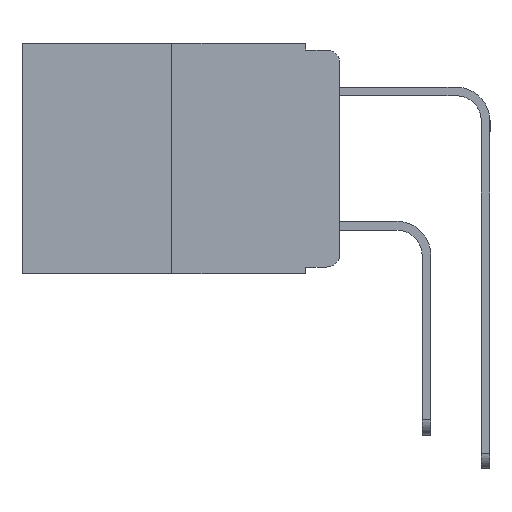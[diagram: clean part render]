
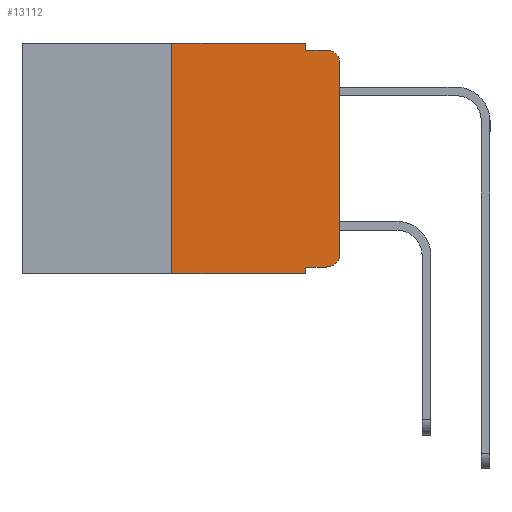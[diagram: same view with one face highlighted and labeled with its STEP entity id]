
A CAD part, left-side view. The second image highlights one B-rep face of the part: STEP entity #13112.
In plain terms, the highlighted planar face has unit normal (-1, 0, 0).
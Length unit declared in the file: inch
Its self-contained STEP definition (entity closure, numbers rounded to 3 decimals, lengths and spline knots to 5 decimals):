
#239 = VERTEX_POINT ( 'NONE', #8575 ) ;
#1704 = VERTEX_POINT ( 'NONE', #5237 ) ;
#1917 = VERTEX_POINT ( 'NONE', #10262 ) ;
#2383 = VECTOR ( 'NONE', #9094, 39.37008 ) ;
#2696 = ORIENTED_EDGE ( 'NONE', *, *, #4232, .T. ) ;
#3039 = LINE ( 'NONE', #15626, #9622 ) ;
#3083 = EDGE_CURVE ( 'NONE', #10547, #7417, #3039, .T. ) ;
#3260 = ORIENTED_EDGE ( 'NONE', *, *, #15916, .T. ) ;
#3425 = ORIENTED_EDGE ( 'NONE', *, *, #4683, .T. ) ;
#3644 = DIRECTION ( 'NONE',  ( 1., 0., 0. ) ) ;
#3712 = VERTEX_POINT ( 'NONE', #8653 ) ;
#3813 = EDGE_CURVE ( 'NONE', #7417, #6223, #8644, .T. ) ;
#3846 = CARTESIAN_POINT ( 'NONE',  ( 0., 0.473, -0.343 ) ) ;
#4232 = EDGE_CURVE ( 'NONE', #1704, #3712, #5195, .T. ) ;
#4366 = CIRCLE ( 'NONE', #16065, 0.02 ) ;
#4436 = CARTESIAN_POINT ( 'NONE',  ( 0., 0.051, 0. ) ) ;
#4580 = VECTOR ( 'NONE', #11531, 39.37008 ) ;
#4683 = EDGE_CURVE ( 'NONE', #10547, #239, #14860, .T. ) ;
#4753 = EDGE_CURVE ( 'NONE', #15833, #10341, #4366, .T. ) ;
#4819 = CIRCLE ( 'NONE', #9872, 0.02 ) ;
#5162 = CARTESIAN_POINT ( 'NONE',  ( 0., 0.02, -0.313 ) ) ;
#5195 = LINE ( 'NONE', #8244, #8019 ) ;
#5237 = CARTESIAN_POINT ( 'NONE',  ( 0., 0.051, -0.333 ) ) ;
#5358 = AXIS2_PLACEMENT_3D ( 'NONE', #11033, #3644, #12258 ) ;
#5512 = DIRECTION ( 'NONE',  ( 0., 0., -1. ) ) ;
#5885 = VECTOR ( 'NONE', #14178, 39.37008 ) ;
#5941 = EDGE_CURVE ( 'NONE', #1704, #239, #6253, .T. ) ;
#6223 = VERTEX_POINT ( 'NONE', #15981 ) ;
#6253 = LINE ( 'NONE', #4436, #5885 ) ;
#6355 = DIRECTION ( 'NONE',  ( 0., 0., -1. ) ) ;
#6383 = DIRECTION ( 'NONE',  ( -1., 0., 0. ) ) ;
#6387 = VECTOR ( 'NONE', #7710, 39.37008 ) ;
#6838 = CARTESIAN_POINT ( 'NONE',  ( 0., 0.02, -0.03 ) ) ;
#7074 = ORIENTED_EDGE ( 'NONE', *, *, #3813, .F. ) ;
#7205 = ORIENTED_EDGE ( 'NONE', *, *, #13690, .F. ) ;
#7300 = DIRECTION ( 'NONE',  ( 0., 0., 1. ) ) ;
#7417 = VERTEX_POINT ( 'NONE', #10091 ) ;
#7422 = EDGE_CURVE ( 'NONE', #1917, #10341, #16097, .T. ) ;
#7710 = DIRECTION ( 'NONE',  ( 0., -1., 0. ) ) ;
#8019 = VECTOR ( 'NONE', #10734, 39.37008 ) ;
#8244 = CARTESIAN_POINT ( 'NONE',  ( 0., 0.051, -0.333 ) ) ;
#8575 = CARTESIAN_POINT ( 'NONE',  ( 0., 0.051, -0.343 ) ) ;
#8619 = LINE ( 'NONE', #9923, #14722 ) ;
#8644 = LINE ( 'NONE', #14735, #2383 ) ;
#8653 = CARTESIAN_POINT ( 'NONE',  ( 0., 0.02, -0.333 ) ) ;
#8747 = DIRECTION ( 'NONE',  ( 0., 0., 1. ) ) ;
#9083 = CARTESIAN_POINT ( 'NONE',  ( 0., 0.051, 0. ) ) ;
#9094 = DIRECTION ( 'NONE',  ( 0., -1., 0. ) ) ;
#9380 = VERTEX_POINT ( 'NONE', #12667 ) ;
#9533 = VECTOR ( 'NONE', #10553, 39.37008 ) ;
#9622 = VECTOR ( 'NONE', #7300, 39.37008 ) ;
#9872 = AXIS2_PLACEMENT_3D ( 'NONE', #5162, #13649, #6355 ) ;
#9923 = CARTESIAN_POINT ( 'NONE',  ( 0., 0., 0. ) ) ;
#10091 = CARTESIAN_POINT ( 'NONE',  ( 0., 0.25, 0. ) ) ;
#10143 = FACE_OUTER_BOUND ( 'NONE', #16066, .T. ) ;
#10262 = CARTESIAN_POINT ( 'NONE',  ( 0., 0.051, -0.01 ) ) ;
#10341 = VERTEX_POINT ( 'NONE', #15782 ) ;
#10547 = VERTEX_POINT ( 'NONE', #13608 ) ;
#10553 = DIRECTION ( 'NONE',  ( 0., -1., 0. ) ) ;
#10734 = DIRECTION ( 'NONE',  ( 0., -1., 0. ) ) ;
#10991 = ORIENTED_EDGE ( 'NONE', *, *, #13216, .T. ) ;
#11033 = CARTESIAN_POINT ( 'NONE',  ( 0., 0.473, 0. ) ) ;
#11037 = CARTESIAN_POINT ( 'NONE',  ( 0., 0., -0.03 ) ) ;
#11122 = LINE ( 'NONE', #9083, #4580 ) ;
#11518 = ORIENTED_EDGE ( 'NONE', *, *, #3083, .F. ) ;
#11531 = DIRECTION ( 'NONE',  ( 0., 0., -1. ) ) ;
#11773 = ORIENTED_EDGE ( 'NONE', *, *, #7422, .F. ) ;
#12258 = DIRECTION ( 'NONE',  ( 0., 0., -1. ) ) ;
#12667 = CARTESIAN_POINT ( 'NONE',  ( 0., 0., -0.313 ) ) ;
#13060 = ORIENTED_EDGE ( 'NONE', *, *, #4753, .T. ) ;
#13112 = ADVANCED_FACE ( 'NONE', ( #10143 ), #14623, .F. ) ;
#13216 = EDGE_CURVE ( 'NONE', #9380, #15833, #8619, .T. ) ;
#13466 = ORIENTED_EDGE ( 'NONE', *, *, #5941, .F. ) ;
#13608 = CARTESIAN_POINT ( 'NONE',  ( 0., 0.25, -0.343 ) ) ;
#13649 = DIRECTION ( 'NONE',  ( -1., 0., 0. ) ) ;
#13690 = EDGE_CURVE ( 'NONE', #6223, #1917, #11122, .T. ) ;
#13767 = CARTESIAN_POINT ( 'NONE',  ( 0., 0.051, -0.01 ) ) ;
#14178 = DIRECTION ( 'NONE',  ( 0., 0., -1. ) ) ;
#14623 = PLANE ( 'NONE',  #5358 ) ;
#14722 = VECTOR ( 'NONE', #8747, 39.37008 ) ;
#14735 = CARTESIAN_POINT ( 'NONE',  ( 0., 0.473, 0. ) ) ;
#14860 = LINE ( 'NONE', #3846, #9533 ) ;
#15626 = CARTESIAN_POINT ( 'NONE',  ( 0., 0.25, 0. ) ) ;
#15782 = CARTESIAN_POINT ( 'NONE',  ( 0., 0.02, -0.01 ) ) ;
#15833 = VERTEX_POINT ( 'NONE', #11037 ) ;
#15916 = EDGE_CURVE ( 'NONE', #3712, #9380, #4819, .T. ) ;
#15981 = CARTESIAN_POINT ( 'NONE',  ( 0., 0.051, 0. ) ) ;
#16065 = AXIS2_PLACEMENT_3D ( 'NONE', #6838, #6383, #5512 ) ;
#16066 = EDGE_LOOP ( 'NONE', ( #10991, #13060, #11773, #7205, #7074, #11518, #3425, #13466, #2696, #3260 ) ) ;
#16097 = LINE ( 'NONE', #13767, #6387 ) ;
